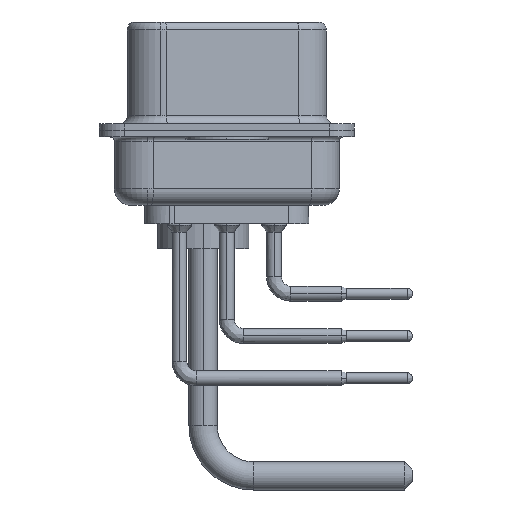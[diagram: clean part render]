
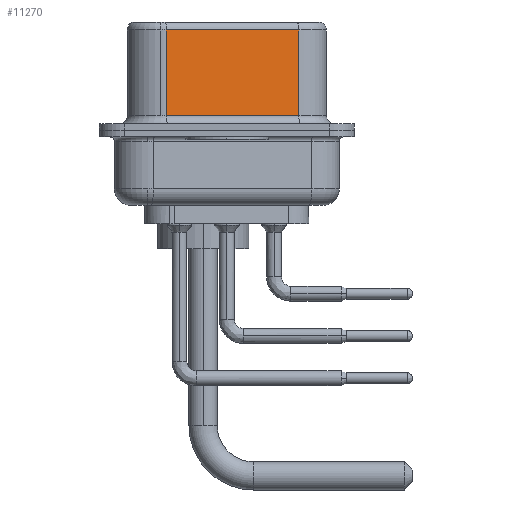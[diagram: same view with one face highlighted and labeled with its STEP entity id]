
A CAD part, left-side view. The second image highlights one B-rep face of the part: STEP entity #11270.
In plain terms, the highlighted planar face has unit normal (-0.985, -0.174, 0).
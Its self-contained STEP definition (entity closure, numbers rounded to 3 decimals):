
#1194 = LINE ( 'NONE', #31604, #25268 ) ;
#3053 = ORIENTED_EDGE ( 'NONE', *, *, #16829, .F. ) ;
#4425 = LINE ( 'NONE', #34668, #9888 ) ;
#5185 = EDGE_CURVE ( 'NONE', #15789, #28069, #24781, .T. ) ;
#5689 = DIRECTION ( 'NONE',  ( -0.174, 0.985, 0. ) ) ;
#7217 = ORIENTED_EDGE ( 'NONE', *, *, #19335, .T. ) ;
#7585 = CARTESIAN_POINT ( 'NONE',  ( 5.132, -4.322, 6.52 ) ) ;
#9888 = VECTOR ( 'NONE', #29650, 1000. ) ;
#10237 = EDGE_CURVE ( 'NONE', #32194, #34254, #4425, .T. ) ;
#11032 = CARTESIAN_POINT ( 'NONE',  ( 3.73, 3.628, 6.02 ) ) ;
#11270 = ADVANCED_FACE ( 'NONE', ( #16841 ), #19199, .F. ) ;
#11607 = CARTESIAN_POINT ( 'NONE',  ( 5.132, -4.322, 6.52 ) ) ;
#13485 = CARTESIAN_POINT ( 'NONE',  ( 5.132, -4.322, 6.02 ) ) ;
#15075 = VECTOR ( 'NONE', #5689, 1000. ) ;
#15415 = CARTESIAN_POINT ( 'NONE',  ( 3.73, 3.628, 0.9 ) ) ;
#15789 = VERTEX_POINT ( 'NONE', #13485 ) ;
#16719 = ORIENTED_EDGE ( 'NONE', *, *, #10237, .T. ) ;
#16829 = EDGE_CURVE ( 'NONE', #15789, #34254, #26513, .T. ) ;
#16841 = FACE_OUTER_BOUND ( 'NONE', #25562, .T. ) ;
#19199 = PLANE ( 'NONE',  #28372 ) ;
#19335 = EDGE_CURVE ( 'NONE', #28069, #32194, #1194, .T. ) ;
#21729 = CARTESIAN_POINT ( 'NONE',  ( 5.132, -4.322, 6.02 ) ) ;
#22618 = DIRECTION ( 'NONE',  ( 0.985, 0.174, 0. ) ) ;
#24781 = LINE ( 'NONE', #21729, #15075 ) ;
#25268 = VECTOR ( 'NONE', #33775, 1000. ) ;
#25562 = EDGE_LOOP ( 'NONE', ( #3053, #32497, #7217, #16719 ) ) ;
#25707 = CARTESIAN_POINT ( 'NONE',  ( 5.132, -4.322, 0.9 ) ) ;
#26513 = LINE ( 'NONE', #7585, #33778 ) ;
#26689 = DIRECTION ( 'NONE',  ( 0., 0., -1. ) ) ;
#28069 = VERTEX_POINT ( 'NONE', #11032 ) ;
#28372 = AXIS2_PLACEMENT_3D ( 'NONE', #11607, #22618, #33610 ) ;
#29650 = DIRECTION ( 'NONE',  ( 0.174, -0.985, 0. ) ) ;
#31604 = CARTESIAN_POINT ( 'NONE',  ( 3.73, 3.628, 6.52 ) ) ;
#32194 = VERTEX_POINT ( 'NONE', #15415 ) ;
#32497 = ORIENTED_EDGE ( 'NONE', *, *, #5185, .T. ) ;
#33610 = DIRECTION ( 'NONE',  ( -0.174, 0.985, 0. ) ) ;
#33775 = DIRECTION ( 'NONE',  ( 0., 0., -1. ) ) ;
#33778 = VECTOR ( 'NONE', #26689, 1000. ) ;
#34254 = VERTEX_POINT ( 'NONE', #25707 ) ;
#34668 = CARTESIAN_POINT ( 'NONE',  ( 5.132, -4.322, 0.9 ) ) ;
